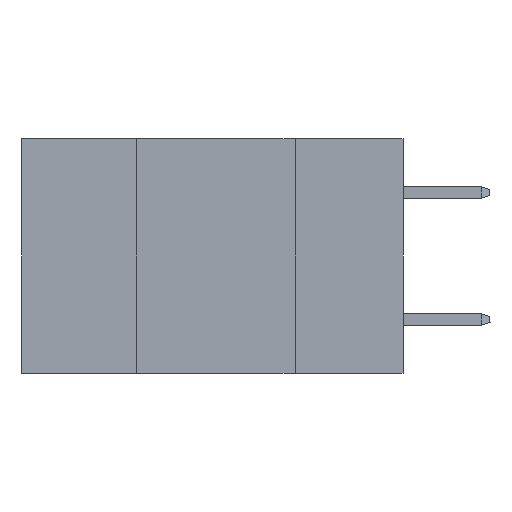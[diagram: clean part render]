
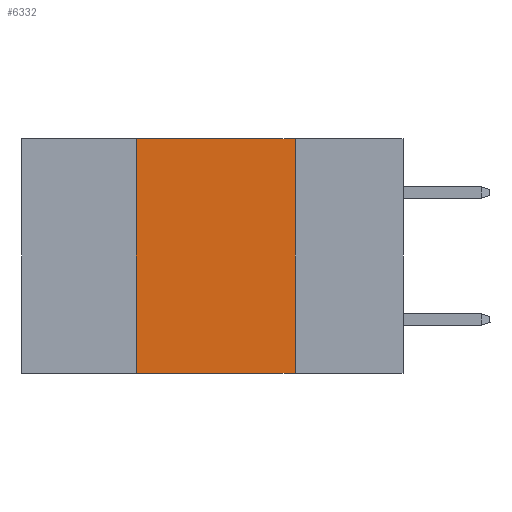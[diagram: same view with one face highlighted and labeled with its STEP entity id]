
A CAD part, left-side view. The second image highlights one B-rep face of the part: STEP entity #6332.
In plain terms, the highlighted planar face has unit normal (-1, 0, 0).
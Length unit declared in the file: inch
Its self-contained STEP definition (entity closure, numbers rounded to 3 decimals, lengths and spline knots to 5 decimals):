
#57 = VERTEX_POINT ( 'NONE', #729 ) ;
#158 = DIRECTION ( 'NONE',  ( 0., 0., -1. ) ) ;
#305 = DIRECTION ( 'NONE',  ( 0., 0., -1. ) ) ;
#729 = CARTESIAN_POINT ( 'NONE',  ( 0., 0.17, -0.37 ) ) ;
#931 = LINE ( 'NONE', #11773, #4101 ) ;
#1033 = CARTESIAN_POINT ( 'NONE',  ( 0., 0.6, -0.37 ) ) ;
#1044 = ORIENTED_EDGE ( 'NONE', *, *, #13628, .F. ) ;
#1194 = CARTESIAN_POINT ( 'NONE',  ( 0., 0.6, 0. ) ) ;
#2066 = EDGE_CURVE ( 'NONE', #5739, #57, #8539, .T. ) ;
#2942 = CARTESIAN_POINT ( 'NONE',  ( 0., 0.17, 0. ) ) ;
#3965 = CARTESIAN_POINT ( 'NONE',  ( 0., 0.42, -0.37 ) ) ;
#4101 = VECTOR ( 'NONE', #6542, 39.37008 ) ;
#5028 = ORIENTED_EDGE ( 'NONE', *, *, #5376, .F. ) ;
#5042 = EDGE_CURVE ( 'NONE', #12948, #57, #7483, .T. ) ;
#5259 = ORIENTED_EDGE ( 'NONE', *, *, #5042, .T. ) ;
#5376 = EDGE_CURVE ( 'NONE', #12948, #13351, #931, .T. ) ;
#5403 = CARTESIAN_POINT ( 'NONE',  ( 0., 0.42, 0. ) ) ;
#5583 = FACE_OUTER_BOUND ( 'NONE', #6908, .T. ) ;
#5739 = VERTEX_POINT ( 'NONE', #2942 ) ;
#6332 = ADVANCED_FACE ( 'NONE', ( #5583 ), #13123, .F. ) ;
#6542 = DIRECTION ( 'NONE',  ( 0., 0., 1. ) ) ;
#6908 = EDGE_LOOP ( 'NONE', ( #9994, #1044, #5028, #5259 ) ) ;
#7483 = LINE ( 'NONE', #1033, #13434 ) ;
#7508 = CARTESIAN_POINT ( 'NONE',  ( 0., 0.17, 0. ) ) ;
#7947 = VECTOR ( 'NONE', #12056, 39.37008 ) ;
#8539 = LINE ( 'NONE', #7508, #10825 ) ;
#9994 = ORIENTED_EDGE ( 'NONE', *, *, #2066, .F. ) ;
#10470 = AXIS2_PLACEMENT_3D ( 'NONE', #1194, #11833, #158 ) ;
#10703 = DIRECTION ( 'NONE',  ( 0., -1., 0. ) ) ;
#10825 = VECTOR ( 'NONE', #305, 39.37008 ) ;
#11080 = CARTESIAN_POINT ( 'NONE',  ( 0., 0.6, 0. ) ) ;
#11773 = CARTESIAN_POINT ( 'NONE',  ( 0., 0.42, 0. ) ) ;
#11833 = DIRECTION ( 'NONE',  ( 1., 0., 0. ) ) ;
#12056 = DIRECTION ( 'NONE',  ( 0., -1., 0. ) ) ;
#12948 = VERTEX_POINT ( 'NONE', #3965 ) ;
#13061 = LINE ( 'NONE', #11080, #7947 ) ;
#13123 = PLANE ( 'NONE',  #10470 ) ;
#13351 = VERTEX_POINT ( 'NONE', #5403 ) ;
#13434 = VECTOR ( 'NONE', #10703, 39.37008 ) ;
#13628 = EDGE_CURVE ( 'NONE', #13351, #5739, #13061, .T. ) ;
